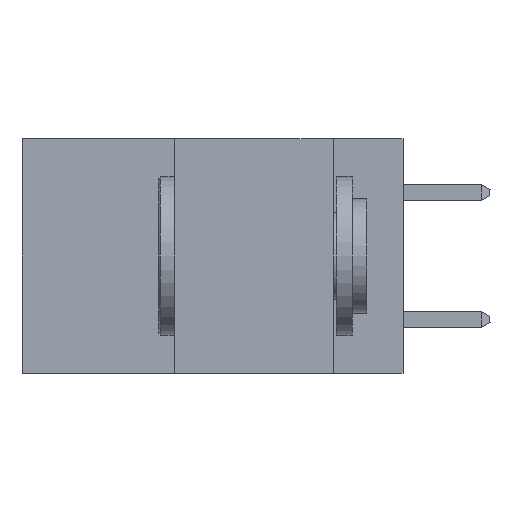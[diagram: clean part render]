
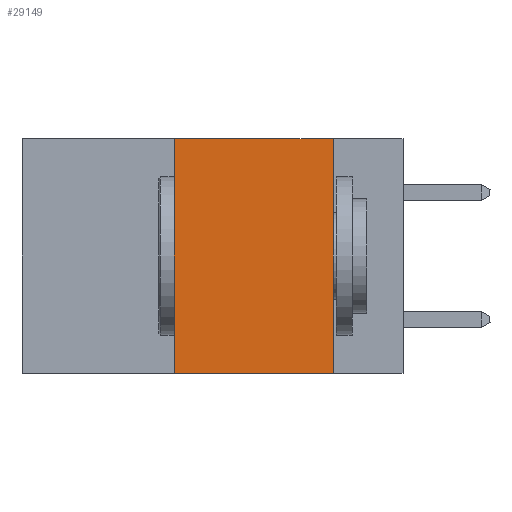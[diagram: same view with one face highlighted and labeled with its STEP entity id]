
A CAD part, left-side view. The second image highlights one B-rep face of the part: STEP entity #29149.
In plain terms, the highlighted planar face has unit normal (-1, 0, 0).
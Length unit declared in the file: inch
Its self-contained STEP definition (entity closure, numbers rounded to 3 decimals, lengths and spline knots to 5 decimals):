
#592 = CARTESIAN_POINT ( 'NONE',  ( 0., 0.11, 0. ) ) ;
#2167 = CARTESIAN_POINT ( 'NONE',  ( 0., 0.11, 0. ) ) ;
#4052 = ORIENTED_EDGE ( 'NONE', *, *, #22288, .F. ) ;
#4671 = ORIENTED_EDGE ( 'NONE', *, *, #10709, .T. ) ;
#5946 = VERTEX_POINT ( 'NONE', #592 ) ;
#6164 = CARTESIAN_POINT ( 'NONE',  ( 0., 0.6, -0.37 ) ) ;
#6869 = EDGE_CURVE ( 'NONE', #28374, #15004, #14795, .T. ) ;
#10397 = DIRECTION ( 'NONE',  ( 0., 0., -1. ) ) ;
#10709 = EDGE_CURVE ( 'NONE', #28374, #13323, #13590, .T. ) ;
#11427 = CARTESIAN_POINT ( 'NONE',  ( 0., 0.36, 0. ) ) ;
#12150 = CARTESIAN_POINT ( 'NONE',  ( 0., 0.11, -0.37 ) ) ;
#13323 = VERTEX_POINT ( 'NONE', #12150 ) ;
#13372 = VECTOR ( 'NONE', #14427, 39.37008 ) ;
#13590 = LINE ( 'NONE', #6164, #28694 ) ;
#13747 = DIRECTION ( 'NONE',  ( 0., 0., -1. ) ) ;
#14427 = DIRECTION ( 'NONE',  ( 0., 0., 1. ) ) ;
#14457 = LINE ( 'NONE', #34083, #25303 ) ;
#14795 = LINE ( 'NONE', #29474, #13372 ) ;
#15004 = VERTEX_POINT ( 'NONE', #11427 ) ;
#16088 = ORIENTED_EDGE ( 'NONE', *, *, #21060, .F. ) ;
#16470 = CARTESIAN_POINT ( 'NONE',  ( 0., 0.6, 0. ) ) ;
#21060 = EDGE_CURVE ( 'NONE', #5946, #13323, #28713, .T. ) ;
#21204 = DIRECTION ( 'NONE',  ( 0., -1., 0. ) ) ;
#22203 = CARTESIAN_POINT ( 'NONE',  ( 0., 0.36, -0.37 ) ) ;
#22288 = EDGE_CURVE ( 'NONE', #15004, #5946, #14457, .T. ) ;
#24875 = DIRECTION ( 'NONE',  ( 0., -1., 0. ) ) ;
#24930 = ORIENTED_EDGE ( 'NONE', *, *, #6869, .F. ) ;
#25303 = VECTOR ( 'NONE', #24875, 39.37008 ) ;
#27756 = VECTOR ( 'NONE', #13747, 39.37008 ) ;
#28374 = VERTEX_POINT ( 'NONE', #22203 ) ;
#28694 = VECTOR ( 'NONE', #21204, 39.37008 ) ;
#28713 = LINE ( 'NONE', #2167, #27756 ) ;
#29149 = ADVANCED_FACE ( 'NONE', ( #31650 ), #34492, .F. ) ;
#29474 = CARTESIAN_POINT ( 'NONE',  ( 0., 0.36, 0. ) ) ;
#31650 = FACE_OUTER_BOUND ( 'NONE', #35920, .T. ) ;
#34083 = CARTESIAN_POINT ( 'NONE',  ( 0., 0.6, 0. ) ) ;
#34236 = DIRECTION ( 'NONE',  ( 1., 0., 0. ) ) ;
#34492 = PLANE ( 'NONE',  #37831 ) ;
#35920 = EDGE_LOOP ( 'NONE', ( #16088, #4052, #24930, #4671 ) ) ;
#37831 = AXIS2_PLACEMENT_3D ( 'NONE', #16470, #34236, #10397 ) ;
